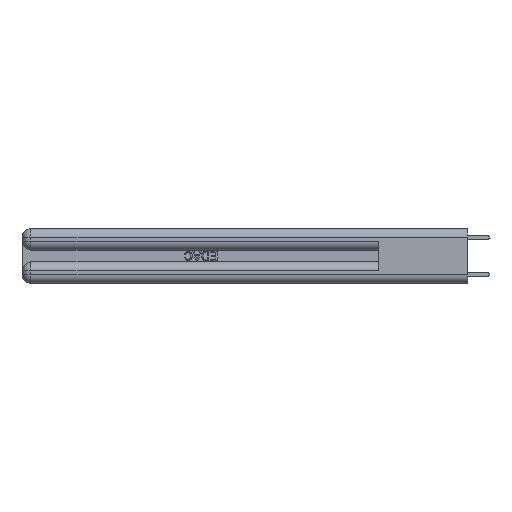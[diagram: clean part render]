
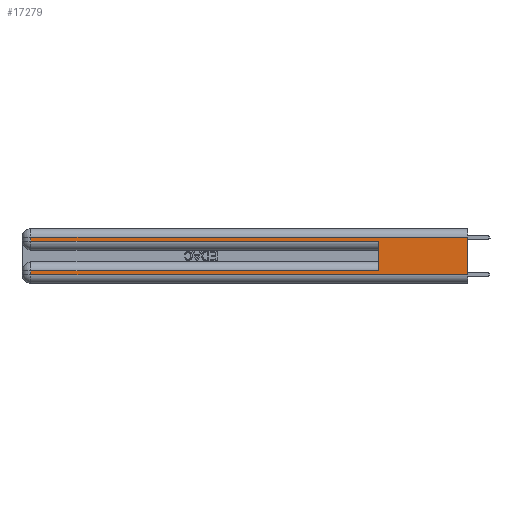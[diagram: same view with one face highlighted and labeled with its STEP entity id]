
A CAD part, left-side view. The second image highlights one B-rep face of the part: STEP entity #17279.
In plain terms, the highlighted planar face has unit normal (-1, 0, 0).
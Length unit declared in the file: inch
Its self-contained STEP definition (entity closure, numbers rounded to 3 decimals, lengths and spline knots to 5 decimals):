
#528 = ORIENTED_EDGE ( 'NONE', *, *, #32262, .T. ) ;
#2125 = CARTESIAN_POINT ( 'NONE',  ( 0., 0.6, 0.285 ) ) ;
#3326 = DIRECTION ( 'NONE',  ( 0., 0., -1. ) ) ;
#3942 = ORIENTED_EDGE ( 'NONE', *, *, #26555, .T. ) ;
#4280 = VECTOR ( 'NONE', #32966, 39.37008 ) ;
#5283 = CARTESIAN_POINT ( 'NONE',  ( 0., 0., 0.31 ) ) ;
#5875 = ORIENTED_EDGE ( 'NONE', *, *, #11193, .T. ) ;
#6054 = CARTESIAN_POINT ( 'NONE',  ( 0., 0.6, 0.085 ) ) ;
#6879 = VERTEX_POINT ( 'NONE', #9084 ) ;
#7423 = LINE ( 'NONE', #8453, #18392 ) ;
#7489 = VERTEX_POINT ( 'NONE', #10693 ) ;
#7691 = VECTOR ( 'NONE', #15527, 39.37008 ) ;
#8453 = CARTESIAN_POINT ( 'NONE',  ( 0., 0., 0.285 ) ) ;
#8742 = CARTESIAN_POINT ( 'NONE',  ( 0., 0.6, 0.145 ) ) ;
#9084 = CARTESIAN_POINT ( 'NONE',  ( 0., 0., 0.31 ) ) ;
#9180 = EDGE_LOOP ( 'NONE', ( #12739, #3942, #528, #34266, #22181, #5875, #33061, #29680 ) ) ;
#9826 = VECTOR ( 'NONE', #3326, 39.37008 ) ;
#9925 = LINE ( 'NONE', #29950, #4280 ) ;
#9965 = CARTESIAN_POINT ( 'NONE',  ( 0., 2.94, 0.06 ) ) ;
#10407 = CARTESIAN_POINT ( 'NONE',  ( 0., 0., 0.06 ) ) ;
#10629 = LINE ( 'NONE', #30644, #24295 ) ;
#10693 = CARTESIAN_POINT ( 'NONE',  ( 0., 2.94, 0.31 ) ) ;
#10865 = VERTEX_POINT ( 'NONE', #9965 ) ;
#11189 = AXIS2_PLACEMENT_3D ( 'NONE', #29726, #18591, #13283 ) ;
#11193 = EDGE_CURVE ( 'NONE', #36026, #32864, #10629, .T. ) ;
#11890 = DIRECTION ( 'NONE',  ( 0., -1., 0. ) ) ;
#12050 = DIRECTION ( 'NONE',  ( 0., 1., 0. ) ) ;
#12739 = ORIENTED_EDGE ( 'NONE', *, *, #19463, .F. ) ;
#13166 = CARTESIAN_POINT ( 'NONE',  ( 0., 0., 0.06 ) ) ;
#13283 = DIRECTION ( 'NONE',  ( 0., 0., -1. ) ) ;
#14084 = CARTESIAN_POINT ( 'NONE',  ( 0., 0., 0.37 ) ) ;
#14142 = EDGE_CURVE ( 'NONE', #36026, #14734, #18037, .T. ) ;
#14734 = VERTEX_POINT ( 'NONE', #2125 ) ;
#15527 = DIRECTION ( 'NONE',  ( 0., 0., -1. ) ) ;
#16919 = VECTOR ( 'NONE', #32770, 39.37008 ) ;
#17279 = ADVANCED_FACE ( 'NONE', ( #26274 ), #27378, .F. ) ;
#17433 = EDGE_CURVE ( 'NONE', #32826, #14734, #7423, .T. ) ;
#18037 = LINE ( 'NONE', #8742, #32905 ) ;
#18392 = VECTOR ( 'NONE', #11890, 39.37008 ) ;
#18591 = DIRECTION ( 'NONE',  ( 1., 0., 0. ) ) ;
#19463 = EDGE_CURVE ( 'NONE', #6879, #30508, #21750, .T. ) ;
#21512 = DIRECTION ( 'NONE',  ( 0., 1., 0. ) ) ;
#21750 = LINE ( 'NONE', #14084, #9826 ) ;
#22033 = DIRECTION ( 'NONE',  ( 0., 0., 1. ) ) ;
#22181 = ORIENTED_EDGE ( 'NONE', *, *, #14142, .F. ) ;
#22584 = CARTESIAN_POINT ( 'NONE',  ( 0., 2.94, 0.285 ) ) ;
#23793 = VECTOR ( 'NONE', #21512, 39.37008 ) ;
#23975 = EDGE_CURVE ( 'NONE', #32864, #10865, #9925, .T. ) ;
#24295 = VECTOR ( 'NONE', #12050, 39.37008 ) ;
#24430 = LINE ( 'NONE', #13166, #16919 ) ;
#24508 = EDGE_CURVE ( 'NONE', #10865, #30508, #24430, .T. ) ;
#25041 = CARTESIAN_POINT ( 'NONE',  ( 0., 2.94, 0.085 ) ) ;
#26274 = FACE_OUTER_BOUND ( 'NONE', #9180, .T. ) ;
#26555 = EDGE_CURVE ( 'NONE', #6879, #7489, #30393, .T. ) ;
#26569 = CARTESIAN_POINT ( 'NONE',  ( 0., 2.94, 0.37 ) ) ;
#27378 = PLANE ( 'NONE',  #11189 ) ;
#29680 = ORIENTED_EDGE ( 'NONE', *, *, #24508, .T. ) ;
#29726 = CARTESIAN_POINT ( 'NONE',  ( 0., 0., 0.37 ) ) ;
#29950 = CARTESIAN_POINT ( 'NONE',  ( 0., 2.94, 0.37 ) ) ;
#30393 = LINE ( 'NONE', #5283, #23793 ) ;
#30508 = VERTEX_POINT ( 'NONE', #10407 ) ;
#30644 = CARTESIAN_POINT ( 'NONE',  ( 0., 0., 0.085 ) ) ;
#32262 = EDGE_CURVE ( 'NONE', #7489, #32826, #32704, .T. ) ;
#32704 = LINE ( 'NONE', #26569, #7691 ) ;
#32770 = DIRECTION ( 'NONE',  ( 0., -1., 0. ) ) ;
#32826 = VERTEX_POINT ( 'NONE', #22584 ) ;
#32864 = VERTEX_POINT ( 'NONE', #25041 ) ;
#32905 = VECTOR ( 'NONE', #22033, 39.37008 ) ;
#32966 = DIRECTION ( 'NONE',  ( 0., 0., -1. ) ) ;
#33061 = ORIENTED_EDGE ( 'NONE', *, *, #23975, .T. ) ;
#34266 = ORIENTED_EDGE ( 'NONE', *, *, #17433, .T. ) ;
#36026 = VERTEX_POINT ( 'NONE', #6054 ) ;
